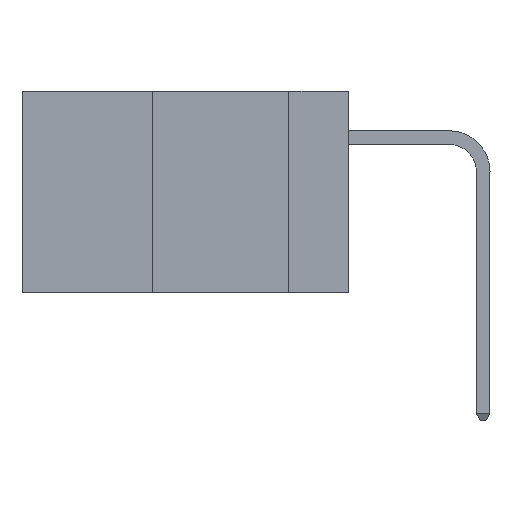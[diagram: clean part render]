
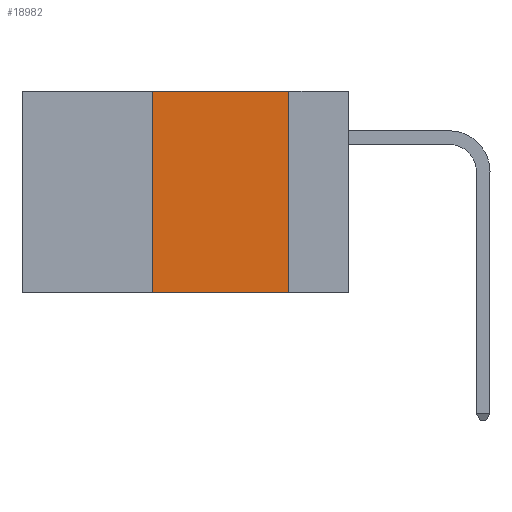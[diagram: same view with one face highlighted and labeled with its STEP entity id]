
A CAD part, left-side view. The second image highlights one B-rep face of the part: STEP entity #18982.
In plain terms, the highlighted planar face has unit normal (-1, 0, 0).
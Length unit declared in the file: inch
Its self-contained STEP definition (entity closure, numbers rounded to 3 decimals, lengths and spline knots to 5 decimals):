
#7 = DIRECTION ( 'NONE',  ( 0., -1., 0. ) ) ;
#1320 = CARTESIAN_POINT ( 'NONE',  ( 0., 0.11, -0.37 ) ) ;
#1385 = ORIENTED_EDGE ( 'NONE', *, *, #12863, .F. ) ;
#1561 = VERTEX_POINT ( 'NONE', #24886 ) ;
#2422 = EDGE_LOOP ( 'NONE', ( #35357, #1385, #6178, #15184 ) ) ;
#3193 = DIRECTION ( 'NONE',  ( 0., 0., -1. ) ) ;
#4140 = AXIS2_PLACEMENT_3D ( 'NONE', #17645, #20653, #3193 ) ;
#5287 = VECTOR ( 'NONE', #17591, 39.37008 ) ;
#6026 = PLANE ( 'NONE',  #4140 ) ;
#6178 = ORIENTED_EDGE ( 'NONE', *, *, #31103, .F. ) ;
#8154 = VERTEX_POINT ( 'NONE', #12169 ) ;
#8880 = DIRECTION ( 'NONE',  ( 0., -1., 0. ) ) ;
#12169 = CARTESIAN_POINT ( 'NONE',  ( 0., 0.36, 0. ) ) ;
#12863 = EDGE_CURVE ( 'NONE', #8154, #1561, #27448, .T. ) ;
#13272 = LINE ( 'NONE', #34572, #35149 ) ;
#14372 = CARTESIAN_POINT ( 'NONE',  ( 0., 0.36, 0. ) ) ;
#15184 = ORIENTED_EDGE ( 'NONE', *, *, #35573, .T. ) ;
#16747 = LINE ( 'NONE', #14372, #23443 ) ;
#17098 = CARTESIAN_POINT ( 'NONE',  ( 0., 0.36, -0.37 ) ) ;
#17567 = CARTESIAN_POINT ( 'NONE',  ( 0., 0.6, 0. ) ) ;
#17591 = DIRECTION ( 'NONE',  ( 0., 0., -1. ) ) ;
#17645 = CARTESIAN_POINT ( 'NONE',  ( 0., 0.6, 0. ) ) ;
#17930 = FACE_OUTER_BOUND ( 'NONE', #2422, .T. ) ;
#18982 = ADVANCED_FACE ( 'NONE', ( #17930 ), #6026, .F. ) ;
#20653 = DIRECTION ( 'NONE',  ( 1., 0., 0. ) ) ;
#23443 = VECTOR ( 'NONE', #34472, 39.37008 ) ;
#24545 = VERTEX_POINT ( 'NONE', #1320 ) ;
#24886 = CARTESIAN_POINT ( 'NONE',  ( 0., 0.11, 0. ) ) ;
#27448 = LINE ( 'NONE', #17567, #34139 ) ;
#28334 = LINE ( 'NONE', #31724, #5287 ) ;
#31103 = EDGE_CURVE ( 'NONE', #36096, #8154, #16747, .T. ) ;
#31724 = CARTESIAN_POINT ( 'NONE',  ( 0., 0.11, 0. ) ) ;
#31812 = EDGE_CURVE ( 'NONE', #1561, #24545, #28334, .T. ) ;
#34139 = VECTOR ( 'NONE', #7, 39.37008 ) ;
#34472 = DIRECTION ( 'NONE',  ( 0., 0., 1. ) ) ;
#34572 = CARTESIAN_POINT ( 'NONE',  ( 0., 0.6, -0.37 ) ) ;
#35149 = VECTOR ( 'NONE', #8880, 39.37008 ) ;
#35357 = ORIENTED_EDGE ( 'NONE', *, *, #31812, .F. ) ;
#35573 = EDGE_CURVE ( 'NONE', #36096, #24545, #13272, .T. ) ;
#36096 = VERTEX_POINT ( 'NONE', #17098 ) ;
